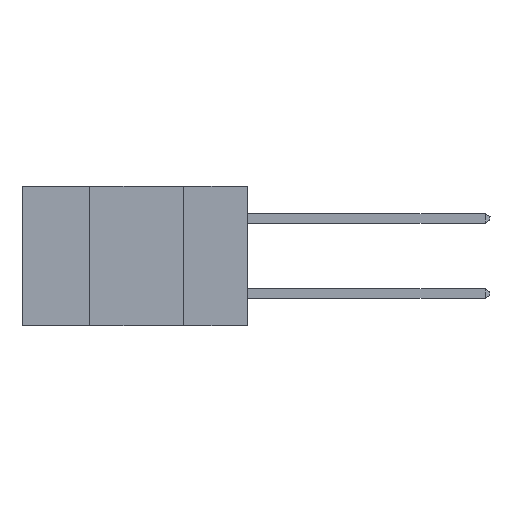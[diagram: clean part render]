
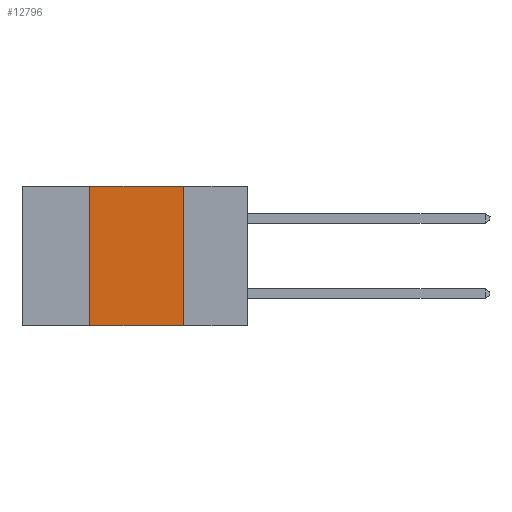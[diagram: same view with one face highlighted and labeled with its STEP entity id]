
A CAD part, left-side view. The second image highlights one B-rep face of the part: STEP entity #12796.
In plain terms, the highlighted planar face has unit normal (-1, 0, 0).
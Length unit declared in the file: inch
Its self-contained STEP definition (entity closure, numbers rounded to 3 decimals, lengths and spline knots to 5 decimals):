
#298 = LINE ( 'NONE', #3914, #18521 ) ;
#1064 = VERTEX_POINT ( 'NONE', #18716 ) ;
#1977 = VECTOR ( 'NONE', #11519, 39.37008 ) ;
#2668 = CARTESIAN_POINT ( 'NONE',  ( 0., 0.42, 0. ) ) ;
#3107 = EDGE_CURVE ( 'NONE', #7067, #20616, #3900, .T. ) ;
#3900 = LINE ( 'NONE', #7035, #23267 ) ;
#3914 = CARTESIAN_POINT ( 'NONE',  ( 0., 0.17, 0. ) ) ;
#4354 = CARTESIAN_POINT ( 'NONE',  ( 0., 0.6, 0. ) ) ;
#4431 = PLANE ( 'NONE',  #14324 ) ;
#5433 = EDGE_CURVE ( 'NONE', #7067, #1064, #12312, .T. ) ;
#6247 = DIRECTION ( 'NONE',  ( 0., 0., -1. ) ) ;
#6955 = DIRECTION ( 'NONE',  ( 0., 0., 1. ) ) ;
#7035 = CARTESIAN_POINT ( 'NONE',  ( 0., 0.42, 0. ) ) ;
#7067 = VERTEX_POINT ( 'NONE', #16033 ) ;
#9379 = ORIENTED_EDGE ( 'NONE', *, *, #22380, .F. ) ;
#9582 = VERTEX_POINT ( 'NONE', #15106 ) ;
#11495 = DIRECTION ( 'NONE',  ( 0., 0., -1. ) ) ;
#11519 = DIRECTION ( 'NONE',  ( 0., -1., 0. ) ) ;
#12312 = LINE ( 'NONE', #14624, #1977 ) ;
#12446 = ORIENTED_EDGE ( 'NONE', *, *, #5433, .T. ) ;
#12796 = ADVANCED_FACE ( 'NONE', ( #21226 ), #4431, .F. ) ;
#14324 = AXIS2_PLACEMENT_3D ( 'NONE', #4354, #19117, #6247 ) ;
#14462 = LINE ( 'NONE', #15427, #19702 ) ;
#14624 = CARTESIAN_POINT ( 'NONE',  ( 0., 0.6, -0.37 ) ) ;
#15106 = CARTESIAN_POINT ( 'NONE',  ( 0., 0.17, 0. ) ) ;
#15427 = CARTESIAN_POINT ( 'NONE',  ( 0., 0.6, 0. ) ) ;
#16033 = CARTESIAN_POINT ( 'NONE',  ( 0., 0.42, -0.37 ) ) ;
#18521 = VECTOR ( 'NONE', #11495, 39.37008 ) ;
#18716 = CARTESIAN_POINT ( 'NONE',  ( 0., 0.17, -0.37 ) ) ;
#19117 = DIRECTION ( 'NONE',  ( 1., 0., 0. ) ) ;
#19274 = EDGE_LOOP ( 'NONE', ( #23342, #9379, #23440, #12446 ) ) ;
#19702 = VECTOR ( 'NONE', #22943, 39.37008 ) ;
#20616 = VERTEX_POINT ( 'NONE', #2668 ) ;
#21226 = FACE_OUTER_BOUND ( 'NONE', #19274, .T. ) ;
#22249 = EDGE_CURVE ( 'NONE', #9582, #1064, #298, .T. ) ;
#22380 = EDGE_CURVE ( 'NONE', #20616, #9582, #14462, .T. ) ;
#22943 = DIRECTION ( 'NONE',  ( 0., -1., 0. ) ) ;
#23267 = VECTOR ( 'NONE', #6955, 39.37008 ) ;
#23342 = ORIENTED_EDGE ( 'NONE', *, *, #22249, .F. ) ;
#23440 = ORIENTED_EDGE ( 'NONE', *, *, #3107, .F. ) ;
